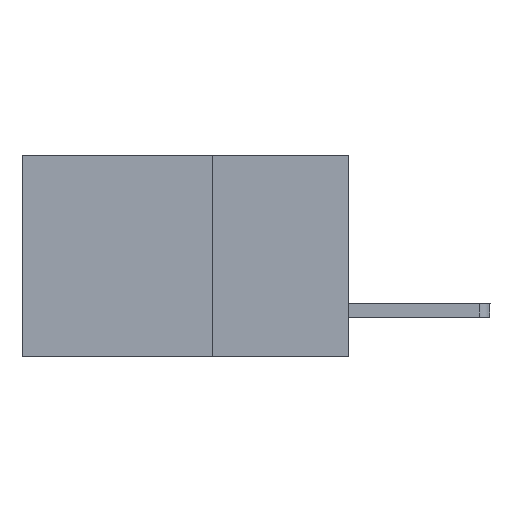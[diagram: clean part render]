
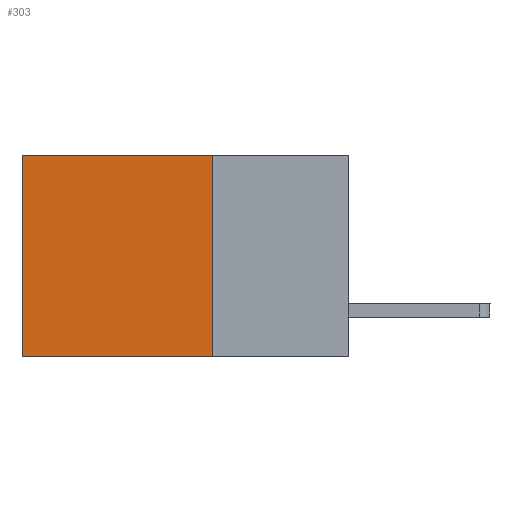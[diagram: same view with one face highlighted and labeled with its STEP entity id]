
A CAD part, left-side view. The second image highlights one B-rep face of the part: STEP entity #303.
In plain terms, the highlighted planar face has unit normal (-1, 0, 0).
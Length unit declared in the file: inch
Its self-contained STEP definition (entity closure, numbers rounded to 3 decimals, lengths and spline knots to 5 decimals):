
#164 = ORIENTED_EDGE ( 'NONE', *, *, #1890, .F. ) ;
#177 = ORIENTED_EDGE ( 'NONE', *, *, #3569, .T. ) ;
#303 = ADVANCED_FACE ( 'NONE', ( #9131 ), #8419, .F. ) ;
#329 = DIRECTION ( 'NONE',  ( 0., 0., -1. ) ) ;
#461 = DIRECTION ( 'NONE',  ( 1., 0., 0. ) ) ;
#971 = DIRECTION ( 'NONE',  ( 0., 1., 0. ) ) ;
#1052 = EDGE_CURVE ( 'NONE', #8177, #5754, #6928, .T. ) ;
#1373 = CARTESIAN_POINT ( 'NONE',  ( 0.2615, 0.25, -0.37 ) ) ;
#1731 = VERTEX_POINT ( 'NONE', #6487 ) ;
#1823 = CARTESIAN_POINT ( 'NONE',  ( 0.2615, 0.6, -0.37 ) ) ;
#1889 = CARTESIAN_POINT ( 'NONE',  ( 0.2615, 0.25, 0. ) ) ;
#1890 = EDGE_CURVE ( 'NONE', #8177, #6553, #8520, .T. ) ;
#2317 = ORIENTED_EDGE ( 'NONE', *, *, #1052, .T. ) ;
#2564 = EDGE_LOOP ( 'NONE', ( #177, #3093, #164, #2317 ) ) ;
#3093 = ORIENTED_EDGE ( 'NONE', *, *, #4501, .F. ) ;
#3569 = EDGE_CURVE ( 'NONE', #5754, #1731, #4041, .T. ) ;
#4041 = LINE ( 'NONE', #1823, #7071 ) ;
#4237 = DIRECTION ( 'NONE',  ( 0., 0., -1. ) ) ;
#4501 = EDGE_CURVE ( 'NONE', #6553, #1731, #7379, .T. ) ;
#4641 = CARTESIAN_POINT ( 'NONE',  ( 0.2615, 0.25, -0.37 ) ) ;
#5187 = CARTESIAN_POINT ( 'NONE',  ( 0.2615, 0.25, -0.37 ) ) ;
#5477 = DIRECTION ( 'NONE',  ( 0., 0., -1. ) ) ;
#5754 = VERTEX_POINT ( 'NONE', #7826 ) ;
#6487 = CARTESIAN_POINT ( 'NONE',  ( 0.2615, 0.6, -0.37 ) ) ;
#6553 = VERTEX_POINT ( 'NONE', #4641 ) ;
#6828 = DIRECTION ( 'NONE',  ( 0., 1., 0. ) ) ;
#6928 = LINE ( 'NONE', #1889, #7907 ) ;
#7071 = VECTOR ( 'NONE', #329, 39.37008 ) ;
#7379 = LINE ( 'NONE', #5187, #9025 ) ;
#7490 = CARTESIAN_POINT ( 'NONE',  ( 0.2615, 0.25, 0. ) ) ;
#7500 = VECTOR ( 'NONE', #4237, 39.37008 ) ;
#7714 = CARTESIAN_POINT ( 'NONE',  ( 0.2615, 0.25, -0.37 ) ) ;
#7826 = CARTESIAN_POINT ( 'NONE',  ( 0.2615, 0.6, 0. ) ) ;
#7907 = VECTOR ( 'NONE', #6828, 39.37008 ) ;
#8177 = VERTEX_POINT ( 'NONE', #7490 ) ;
#8419 = PLANE ( 'NONE',  #8786 ) ;
#8520 = LINE ( 'NONE', #1373, #7500 ) ;
#8786 = AXIS2_PLACEMENT_3D ( 'NONE', #7714, #461, #5477 ) ;
#9025 = VECTOR ( 'NONE', #971, 39.37008 ) ;
#9131 = FACE_OUTER_BOUND ( 'NONE', #2564, .T. ) ;
